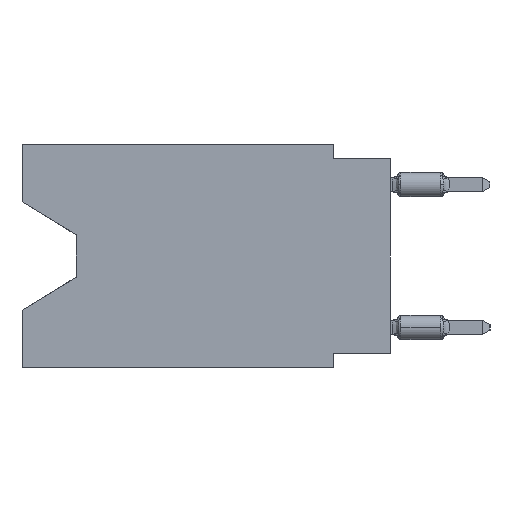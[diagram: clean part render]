
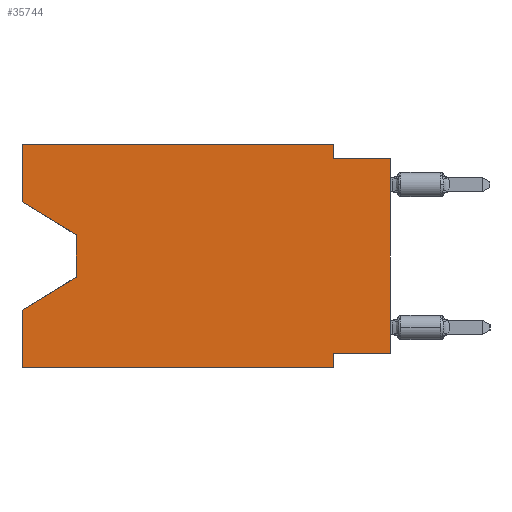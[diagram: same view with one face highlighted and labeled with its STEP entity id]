
A CAD part, left-side view. The second image highlights one B-rep face of the part: STEP entity #35744.
In plain terms, the highlighted planar face has unit normal (-1, 0, 0).
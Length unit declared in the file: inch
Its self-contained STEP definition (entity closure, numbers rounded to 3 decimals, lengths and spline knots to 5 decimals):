
#1292 = DIRECTION ( 'NONE',  ( 0., 0., 1. ) ) ;
#1700 = LINE ( 'NONE', #7957, #6081 ) ;
#1705 = EDGE_CURVE ( 'NONE', #37245, #33795, #23457, .T. ) ;
#2152 = VECTOR ( 'NONE', #30044, 39.37008 ) ;
#2189 = LINE ( 'NONE', #37401, #25172 ) ;
#2707 = EDGE_CURVE ( 'NONE', #23099, #27297, #37240, .T. ) ;
#3866 = CARTESIAN_POINT ( 'NONE',  ( 0., 0.1, -0.39 ) ) ;
#5100 = VECTOR ( 'NONE', #7753, 39.37008 ) ;
#5450 = EDGE_CURVE ( 'NONE', #14845, #22775, #16662, .T. ) ;
#6081 = VECTOR ( 'NONE', #1292, 39.37008 ) ;
#6548 = EDGE_CURVE ( 'NONE', #35435, #32170, #2189, .T. ) ;
#7277 = DIRECTION ( 'NONE',  ( 0., 1., 0. ) ) ;
#7374 = CARTESIAN_POINT ( 'NONE',  ( 0., 0.645, 0. ) ) ;
#7477 = ORIENTED_EDGE ( 'NONE', *, *, #1705, .F. ) ;
#7530 = LINE ( 'NONE', #32964, #2152 ) ;
#7753 = DIRECTION ( 'NONE',  ( 0., 0., -1. ) ) ;
#7957 = CARTESIAN_POINT ( 'NONE',  ( 0., 0.645, 0. ) ) ;
#8884 = DIRECTION ( 'NONE',  ( 0., -0.855, -0.519 ) ) ;
#8927 = CARTESIAN_POINT ( 'NONE',  ( 0., 0.645, -0.39 ) ) ;
#9468 = CARTESIAN_POINT ( 'NONE',  ( 0., 0.55, -0.158 ) ) ;
#9758 = VECTOR ( 'NONE', #37389, 39.37008 ) ;
#9879 = CARTESIAN_POINT ( 'NONE',  ( 0., 0.645, 0. ) ) ;
#10491 = CARTESIAN_POINT ( 'NONE',  ( 0., 0.1, -0.39 ) ) ;
#12079 = FACE_OUTER_BOUND ( 'NONE', #35176, .T. ) ;
#12505 = DIRECTION ( 'NONE',  ( 1., 0., 0. ) ) ;
#12540 = VERTEX_POINT ( 'NONE', #29933 ) ;
#12641 = EDGE_CURVE ( 'NONE', #23850, #34916, #40549, .T. ) ;
#12840 = VECTOR ( 'NONE', #23440, 39.37008 ) ;
#13620 = LINE ( 'NONE', #7374, #25035 ) ;
#14204 = EDGE_CURVE ( 'NONE', #12540, #34916, #1700, .T. ) ;
#14748 = EDGE_CURVE ( 'NONE', #12540, #24027, #34563, .T. ) ;
#14845 = VERTEX_POINT ( 'NONE', #35585 ) ;
#15014 = PLANE ( 'NONE',  #26425 ) ;
#15081 = CARTESIAN_POINT ( 'NONE',  ( 0., 0.645, -0.10025 ) ) ;
#15318 = CARTESIAN_POINT ( 'NONE',  ( 0., 0.645, -0.28975 ) ) ;
#16459 = CARTESIAN_POINT ( 'NONE',  ( 0., 0., -0.365 ) ) ;
#16571 = CARTESIAN_POINT ( 'NONE',  ( 0., 0.1, -0.365 ) ) ;
#16662 = LINE ( 'NONE', #16459, #25707 ) ;
#16957 = ORIENTED_EDGE ( 'NONE', *, *, #14204, .F. ) ;
#16964 = DIRECTION ( 'NONE',  ( 0., 0., 1. ) ) ;
#16974 = CARTESIAN_POINT ( 'NONE',  ( 0., 0., 0. ) ) ;
#17213 = ORIENTED_EDGE ( 'NONE', *, *, #14748, .T. ) ;
#17414 = ORIENTED_EDGE ( 'NONE', *, *, #22973, .T. ) ;
#17785 = EDGE_CURVE ( 'NONE', #33795, #35435, #7530, .T. ) ;
#18132 = ORIENTED_EDGE ( 'NONE', *, *, #23900, .T. ) ;
#18598 = ORIENTED_EDGE ( 'NONE', *, *, #17785, .F. ) ;
#18749 = ORIENTED_EDGE ( 'NONE', *, *, #12641, .T. ) ;
#19043 = ORIENTED_EDGE ( 'NONE', *, *, #31603, .F. ) ;
#20997 = VECTOR ( 'NONE', #32824, 39.37008 ) ;
#21277 = CARTESIAN_POINT ( 'NONE',  ( 0., 0.645, 0. ) ) ;
#21652 = DIRECTION ( 'NONE',  ( 0., -1., 0. ) ) ;
#22193 = DIRECTION ( 'NONE',  ( 0., 0., -1. ) ) ;
#22748 = VECTOR ( 'NONE', #21652, 39.37008 ) ;
#22775 = VERTEX_POINT ( 'NONE', #16571 ) ;
#22973 = EDGE_CURVE ( 'NONE', #14845, #32170, #33413, .T. ) ;
#23099 = VERTEX_POINT ( 'NONE', #15081 ) ;
#23440 = DIRECTION ( 'NONE',  ( 0., 0., 1. ) ) ;
#23457 = LINE ( 'NONE', #29720, #20997 ) ;
#23850 = VERTEX_POINT ( 'NONE', #25331 ) ;
#23900 = EDGE_CURVE ( 'NONE', #27297, #23850, #31183, .T. ) ;
#24027 = VERTEX_POINT ( 'NONE', #3866 ) ;
#24697 = CARTESIAN_POINT ( 'NONE',  ( 0., 0.55, -0.232 ) ) ;
#25035 = VECTOR ( 'NONE', #16964, 39.37008 ) ;
#25172 = VECTOR ( 'NONE', #27431, 39.37008 ) ;
#25331 = CARTESIAN_POINT ( 'NONE',  ( 0., 0.55, -0.232 ) ) ;
#25707 = VECTOR ( 'NONE', #7277, 39.37008 ) ;
#26425 = AXIS2_PLACEMENT_3D ( 'NONE', #21277, #12505, #34178 ) ;
#27297 = VERTEX_POINT ( 'NONE', #29951 ) ;
#27431 = DIRECTION ( 'NONE',  ( 0., -1., 0. ) ) ;
#28264 = CARTESIAN_POINT ( 'NONE',  ( 0., 0., -0.025 ) ) ;
#29276 = ORIENTED_EDGE ( 'NONE', *, *, #2707, .T. ) ;
#29720 = CARTESIAN_POINT ( 'NONE',  ( 0., 0.645, 0. ) ) ;
#29933 = CARTESIAN_POINT ( 'NONE',  ( 0., 0.645, -0.39 ) ) ;
#29951 = CARTESIAN_POINT ( 'NONE',  ( 0., 0.55, -0.158 ) ) ;
#30012 = ORIENTED_EDGE ( 'NONE', *, *, #35062, .F. ) ;
#30044 = DIRECTION ( 'NONE',  ( 0., 0., -1. ) ) ;
#30660 = ORIENTED_EDGE ( 'NONE', *, *, #6548, .F. ) ;
#31183 = LINE ( 'NONE', #9468, #38764 ) ;
#31603 = EDGE_CURVE ( 'NONE', #22775, #24027, #38816, .T. ) ;
#32170 = VERTEX_POINT ( 'NONE', #28264 ) ;
#32824 = DIRECTION ( 'NONE',  ( 0., -1., 0. ) ) ;
#32964 = CARTESIAN_POINT ( 'NONE',  ( 0., 0.1, 0. ) ) ;
#33413 = LINE ( 'NONE', #16974, #12840 ) ;
#33795 = VERTEX_POINT ( 'NONE', #38205 ) ;
#34178 = DIRECTION ( 'NONE',  ( 0., 0., -1. ) ) ;
#34563 = LINE ( 'NONE', #8927, #22748 ) ;
#34916 = VERTEX_POINT ( 'NONE', #15318 ) ;
#35062 = EDGE_CURVE ( 'NONE', #23099, #37245, #13620, .T. ) ;
#35176 = EDGE_LOOP ( 'NONE', ( #29276, #18132, #18749, #16957, #17213, #19043, #38916, #17414, #30660, #18598, #7477, #30012 ) ) ;
#35435 = VERTEX_POINT ( 'NONE', #35445 ) ;
#35445 = CARTESIAN_POINT ( 'NONE',  ( 0., 0.1, -0.025 ) ) ;
#35585 = CARTESIAN_POINT ( 'NONE',  ( 0., 0., -0.365 ) ) ;
#35744 = ADVANCED_FACE ( 'NONE', ( #12079 ), #15014, .F. ) ;
#37240 = LINE ( 'NONE', #40164, #40528 ) ;
#37245 = VERTEX_POINT ( 'NONE', #9879 ) ;
#37389 = DIRECTION ( 'NONE',  ( 0., 0.855, -0.519 ) ) ;
#37401 = CARTESIAN_POINT ( 'NONE',  ( 0., 0., -0.025 ) ) ;
#38205 = CARTESIAN_POINT ( 'NONE',  ( 0., 0.1, 0. ) ) ;
#38764 = VECTOR ( 'NONE', #22193, 39.37008 ) ;
#38816 = LINE ( 'NONE', #10491, #5100 ) ;
#38916 = ORIENTED_EDGE ( 'NONE', *, *, #5450, .F. ) ;
#40164 = CARTESIAN_POINT ( 'NONE',  ( 0., 0.645, -0.10025 ) ) ;
#40528 = VECTOR ( 'NONE', #8884, 39.37008 ) ;
#40549 = LINE ( 'NONE', #24697, #9758 ) ;
